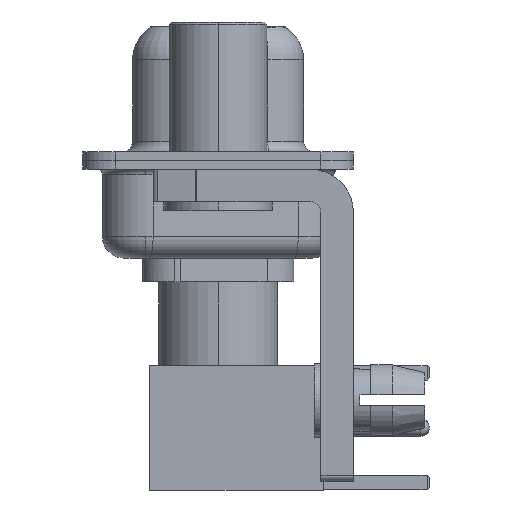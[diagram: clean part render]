
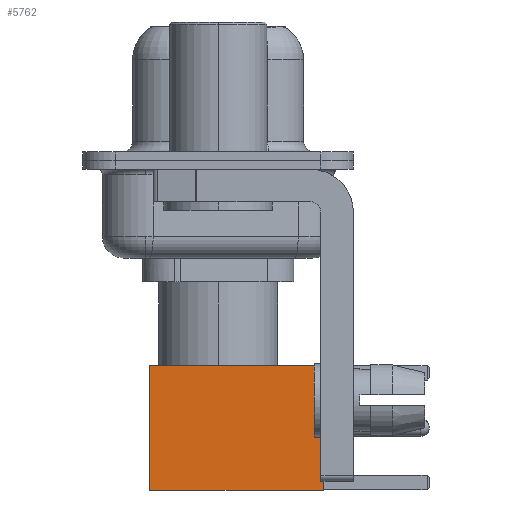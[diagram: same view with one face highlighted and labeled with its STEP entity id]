
A CAD part, left-side view. The second image highlights one B-rep face of the part: STEP entity #5762.
In plain terms, the highlighted face is planar.
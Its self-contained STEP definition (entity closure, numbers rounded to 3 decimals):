
#1541 = LINE ( 'NONE', #19051, #4904 ) ;
#2224 = AXIS2_PLACEMENT_3D ( 'NONE', #20997, #3631, #3746 ) ;
#3250 = VECTOR ( 'NONE', #15892, 1000. ) ;
#3531 = EDGE_CURVE ( 'NONE', #19331, #18245, #10733, .T. ) ;
#3631 = DIRECTION ( 'NONE',  ( 0., 1., 0. ) ) ;
#3696 = CARTESIAN_POINT ( 'NONE',  ( -2.875, 2.875, 0. ) ) ;
#3746 = DIRECTION ( 'NONE',  ( 0., 0., 1. ) ) ;
#4904 = VECTOR ( 'NONE', #10655, 1000. ) ;
#5486 = FACE_OUTER_BOUND ( 'NONE', #7221, .T. ) ;
#5762 = ADVANCED_FACE ( 'NONE', ( #5486 ), #15829, .T. ) ;
#6319 = ORIENTED_EDGE ( 'NONE', *, *, #10466, .F. ) ;
#6421 = CARTESIAN_POINT ( 'NONE',  ( 2.875, 2.875, 8. ) ) ;
#6453 = VECTOR ( 'NONE', #10362, 1000. ) ;
#7221 = EDGE_LOOP ( 'NONE', ( #16217, #13366, #16029, #6319 ) ) ;
#8919 = DIRECTION ( 'NONE',  ( -1., 0., 0. ) ) ;
#10300 = EDGE_CURVE ( 'NONE', #20320, #18245, #1541, .T. ) ;
#10362 = DIRECTION ( 'NONE',  ( 0., 0., -1. ) ) ;
#10466 = EDGE_CURVE ( 'NONE', #11208, #19331, #18244, .T. ) ;
#10655 = DIRECTION ( 'NONE',  ( -1., 0., 0. ) ) ;
#10733 = LINE ( 'NONE', #3696, #3250 ) ;
#11208 = VERTEX_POINT ( 'NONE', #6421 ) ;
#12257 = VECTOR ( 'NONE', #8919, 1000. ) ;
#12304 = EDGE_CURVE ( 'NONE', #11208, #20320, #15418, .T. ) ;
#12552 = CARTESIAN_POINT ( 'NONE',  ( -2.875, 2.875, 8. ) ) ;
#13366 = ORIENTED_EDGE ( 'NONE', *, *, #10300, .T. ) ;
#15418 = LINE ( 'NONE', #17375, #6453 ) ;
#15829 = PLANE ( 'NONE',  #2224 ) ;
#15892 = DIRECTION ( 'NONE',  ( 0., 0., -1. ) ) ;
#16029 = ORIENTED_EDGE ( 'NONE', *, *, #3531, .F. ) ;
#16157 = CARTESIAN_POINT ( 'NONE',  ( 0., 2.875, 8. ) ) ;
#16217 = ORIENTED_EDGE ( 'NONE', *, *, #12304, .T. ) ;
#17375 = CARTESIAN_POINT ( 'NONE',  ( 2.875, 2.875, 0. ) ) ;
#18244 = LINE ( 'NONE', #16157, #12257 ) ;
#18245 = VERTEX_POINT ( 'NONE', #20482 ) ;
#19051 = CARTESIAN_POINT ( 'NONE',  ( 0., 2.875, 0. ) ) ;
#19331 = VERTEX_POINT ( 'NONE', #12552 ) ;
#20320 = VERTEX_POINT ( 'NONE', #20994 ) ;
#20482 = CARTESIAN_POINT ( 'NONE',  ( -2.875, 2.875, 0. ) ) ;
#20994 = CARTESIAN_POINT ( 'NONE',  ( 2.875, 2.875, 0. ) ) ;
#20997 = CARTESIAN_POINT ( 'NONE',  ( 2.875, 2.875, 0. ) ) ;
